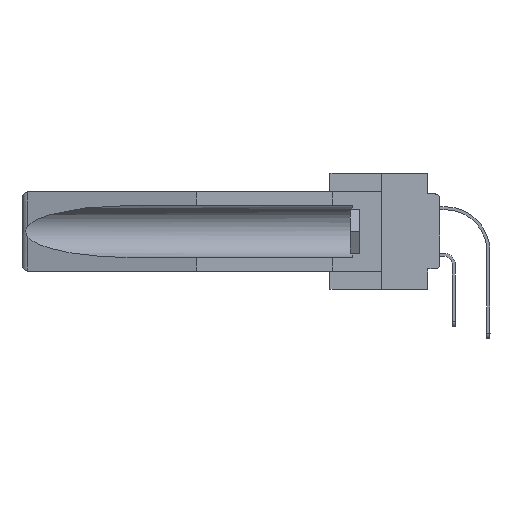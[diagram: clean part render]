
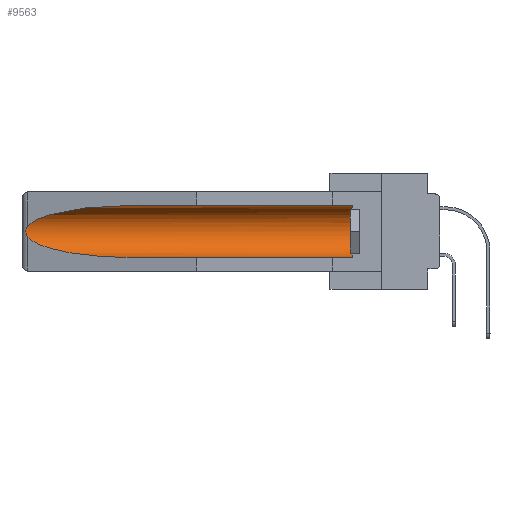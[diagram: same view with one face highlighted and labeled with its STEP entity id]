
A CAD part, left-side view. The second image highlights one B-rep face of the part: STEP entity #9563.
In plain terms, the highlighted cylindrical face has radius 2.857 mm (diameter 5.715 mm), a partial arc.
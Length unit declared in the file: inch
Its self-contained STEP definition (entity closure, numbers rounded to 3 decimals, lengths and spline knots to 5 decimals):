
#603 = CARTESIAN_POINT ( 'NONE',  ( 0.2675, 1.53308, -0.17534 ) ) ;
#665 = CARTESIAN_POINT ( 'NONE',  ( 0.155, -0.30754, -0.059 ) ) ;
#1283 = ORIENTED_EDGE ( 'NONE', *, *, #7804, .T. ) ;
#1695 = CARTESIAN_POINT ( 'NONE',  ( 0.155, -0.30754, -0.1715 ) ) ;
#2059 = DIRECTION ( 'NONE',  ( 0., 0., 1. ) ) ;
#2758 = CARTESIAN_POINT ( 'NONE',  ( 0.26537, 1.52718, -0.19328 ) ) ;
#3113 = CARTESIAN_POINT ( 'NONE',  ( 0.26654, 1.53092, -0.15636 ) ) ;
#3209 = ORIENTED_EDGE ( 'NONE', *, *, #16706, .F. ) ;
#3618 = DIRECTION ( 'NONE',  ( 0., -1., 0. ) ) ;
#3709 = ORIENTED_EDGE ( 'NONE', *, *, #33466, .T. ) ;
#3869 = VERTEX_POINT ( 'NONE', #12504 ) ;
#4730 = LINE ( 'NONE', #13067, #28467 ) ;
#5431 = CARTESIAN_POINT ( 'NONE',  ( 0.2675, 1.53308, -0.16763 ) ) ;
#5951 = CARTESIAN_POINT ( 'NONE',  ( 0.26537, 1.52718, -0.14972 ) ) ;
#6236 = VERTEX_POINT ( 'NONE', #7179 ) ;
#6622 = CARTESIAN_POINT ( 'NONE',  ( 0.25451, 1.48313, -0.24835 ) ) ;
#6783 = DIRECTION ( 'NONE',  ( 0., 0., 1. ) ) ;
#6789 = CARTESIAN_POINT ( 'NONE',  ( 0.26537, 1.52718, -0.19328 ) ) ;
#6824 = ORIENTED_EDGE ( 'NONE', *, *, #30162, .T. ) ;
#7179 = CARTESIAN_POINT ( 'NONE',  ( 0.155, 1.07973, -0.284 ) ) ;
#7804 = EDGE_CURVE ( 'NONE', #10333, #25634, #16722, .T. ) ;
#7838 = VERTEX_POINT ( 'NONE', #17619 ) ;
#8604 = CARTESIAN_POINT ( 'NONE',  ( 0.26597, 1.5296, -0.19026 ) ) ;
#9007 = LINE ( 'NONE', #665, #14733 ) ;
#9366 =( BOUNDED_CURVE ( )  B_SPLINE_CURVE ( 3, ( #6789, #6622, #33678, #9618 ),
 .UNSPECIFIED., .F., .F. ) 
 B_SPLINE_CURVE_WITH_KNOTS ( ( 4, 4 ),
 ( 0.1948, 1.5708 ),
 .UNSPECIFIED. ) 
 CURVE ( )  GEOMETRIC_REPRESENTATION_ITEM ( )  RATIONAL_B_SPLINE_CURVE ( ( 1., 0.848, 0.848, 1. ) ) 
 REPRESENTATION_ITEM ( '' )  );
#9563 = ADVANCED_FACE ( 'NONE', ( #26056 ), #26238, .F. ) ;
#9618 = CARTESIAN_POINT ( 'NONE',  ( 0.155, 1.07973, -0.284 ) ) ;
#10333 = VERTEX_POINT ( 'NONE', #25970 ) ;
#11443 = CARTESIAN_POINT ( 'NONE',  ( 0.26597, 1.52961, -0.15275 ) ) ;
#12482 = EDGE_LOOP ( 'NONE', ( #31370, #31233, #3709, #3209, #1283, #6824 ) ) ;
#12504 = CARTESIAN_POINT ( 'NONE',  ( 0.155, 1.07973, -0.059 ) ) ;
#13067 = CARTESIAN_POINT ( 'NONE',  ( 0.155, -0.30754, -0.284 ) ) ;
#14650 = CARTESIAN_POINT ( 'NONE',  ( 0.21114, 1.30732, -0.059 ) ) ;
#14733 = VECTOR ( 'NONE', #30552, 39.37008 ) ;
#14973 = CARTESIAN_POINT ( 'NONE',  ( 0.155, 0.126, -0.1715 ) ) ;
#15544 = CARTESIAN_POINT ( 'NONE',  ( 0.155, 0.126, -0.059 ) ) ;
#15875 = CARTESIAN_POINT ( 'NONE',  ( 0.26537, 1.52718, -0.19328 ) ) ;
#16706 = EDGE_CURVE ( 'NONE', #10333, #6236, #4730, .T. ) ;
#16722 = CIRCLE ( 'NONE', #18405, 0.1125 ) ;
#17619 = CARTESIAN_POINT ( 'NONE',  ( 0.26537, 1.52718, -0.14972 ) ) ;
#18405 = AXIS2_PLACEMENT_3D ( 'NONE', #14973, #3618, #6783 ) ;
#19465 = CARTESIAN_POINT ( 'NONE',  ( 0.25451, 1.48313, -0.09465 ) ) ;
#19741 = VERTEX_POINT ( 'NONE', #15875 ) ;
#20959 = B_SPLINE_CURVE_WITH_KNOTS ( 'NONE', 3,
 ( #5951, #11443, #3113, #32814, #5431, #603, #26949, #27120, #8604, #2758 ),
 .UNSPECIFIED., .F., .F.,
 ( 4, 2, 2, 2, 4 ),
 ( 0., 0.00029, 0.00058, 0.00087, 0.00117 ),
 .UNSPECIFIED. ) ;
#23393 = DIRECTION ( 'NONE',  ( 0., 1., 0. ) ) ;
#25332 = CARTESIAN_POINT ( 'NONE',  ( 0.26537, 1.52718, -0.14972 ) ) ;
#25634 = VERTEX_POINT ( 'NONE', #15544 ) ;
#25970 = CARTESIAN_POINT ( 'NONE',  ( 0.155, 0.126, -0.284 ) ) ;
#26056 = FACE_OUTER_BOUND ( 'NONE', #12482, .T. ) ;
#26238 = CYLINDRICAL_SURFACE ( 'NONE', #29896, 0.1125 ) ;
#26949 = CARTESIAN_POINT ( 'NONE',  ( 0.2673, 1.53269, -0.17917 ) ) ;
#27120 = CARTESIAN_POINT ( 'NONE',  ( 0.26655, 1.53094, -0.18657 ) ) ;
#28366 = EDGE_CURVE ( 'NONE', #7838, #19741, #20959, .T. ) ;
#28467 = VECTOR ( 'NONE', #31752, 39.37008 ) ;
#29896 = AXIS2_PLACEMENT_3D ( 'NONE', #1695, #23393, #2059 ) ;
#30162 = EDGE_CURVE ( 'NONE', #25634, #3869, #9007, .T. ) ;
#30552 = DIRECTION ( 'NONE',  ( 0., 1., 0. ) ) ;
#30555 = EDGE_CURVE ( 'NONE', #3869, #7838, #34619, .T. ) ;
#31233 = ORIENTED_EDGE ( 'NONE', *, *, #28366, .T. ) ;
#31370 = ORIENTED_EDGE ( 'NONE', *, *, #30555, .T. ) ;
#31752 = DIRECTION ( 'NONE',  ( 0., 1., 0. ) ) ;
#32814 = CARTESIAN_POINT ( 'NONE',  ( 0.2673, 1.5327, -0.16383 ) ) ;
#33466 = EDGE_CURVE ( 'NONE', #19741, #6236, #9366, .T. ) ;
#33678 = CARTESIAN_POINT ( 'NONE',  ( 0.21114, 1.30732, -0.284 ) ) ;
#33697 = CARTESIAN_POINT ( 'NONE',  ( 0.155, 1.07973, -0.059 ) ) ;
#34619 =( BOUNDED_CURVE ( )  B_SPLINE_CURVE ( 3, ( #33697, #14650, #19465, #25332 ),
 .UNSPECIFIED., .F., .F. ) 
 B_SPLINE_CURVE_WITH_KNOTS ( ( 4, 4 ),
 ( 4.71239, 6.08839 ),
 .UNSPECIFIED. ) 
 CURVE ( )  GEOMETRIC_REPRESENTATION_ITEM ( )  RATIONAL_B_SPLINE_CURVE ( ( 1., 0.848, 0.848, 1. ) ) 
 REPRESENTATION_ITEM ( '' )  );
